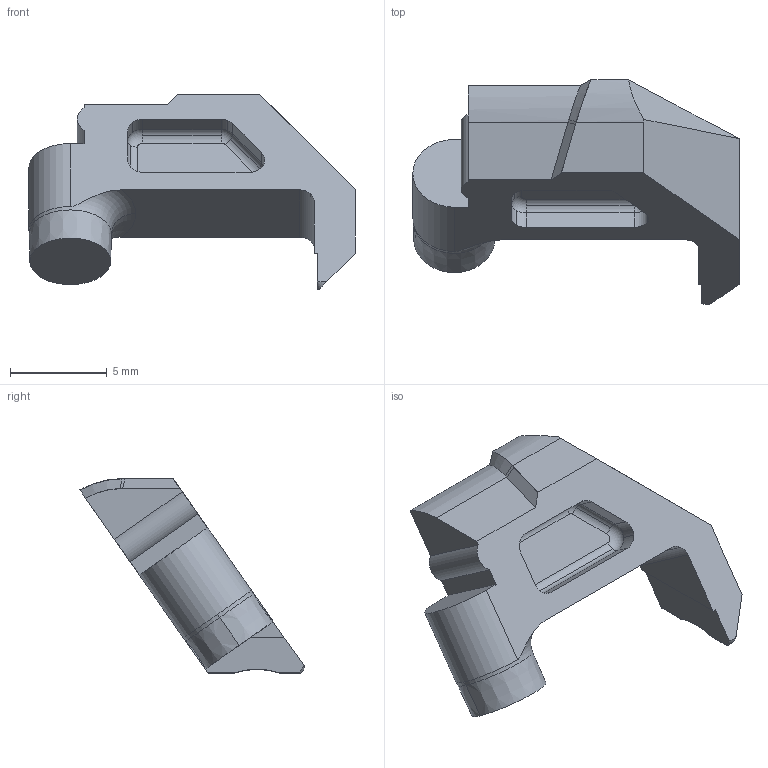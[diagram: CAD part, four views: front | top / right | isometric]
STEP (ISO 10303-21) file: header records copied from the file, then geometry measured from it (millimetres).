
FILE_DESCRIPTION (( 'STEP AP214' ), '1' );
FILE_NAME ('Extractor.step', '2014-07-30T19:45:42', ( 'WarFairy' ), ( '' ), 'SwSTEP 2.0', 'SolidWorks 2013', '' );
FILE_SCHEMA (( 'AUTOMOTIVE_DESIGN' ));
Length unit declared in the file: millimetre
Products named in the file (1): Extractor
Bounding box: 16.87 x 11.59 x 10.06 mm (x, y, z)
Volume: 383.5 mm3; surface area: 516.6 mm2
Topology: 1 solids, 1 shells, 92 faces, 242 edges, 154 vertices
Faces by surface type: cylinder 48, plane 28, torus 11, cone 3, bspline 2
Entity records: 2980 total; most frequent: CARTESIAN_POINT 640, DIRECTION 504, ORIENTED_EDGE 484, EDGE_CURVE 242, AXIS2_PLACEMENT_3D 192, VERTEX_POINT 154, VECTOR 120, LINE 120
